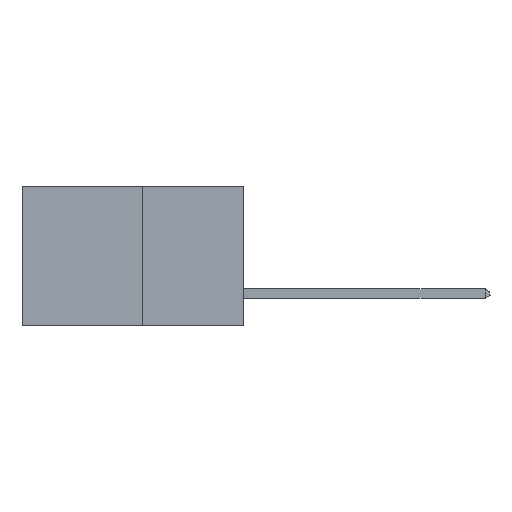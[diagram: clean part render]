
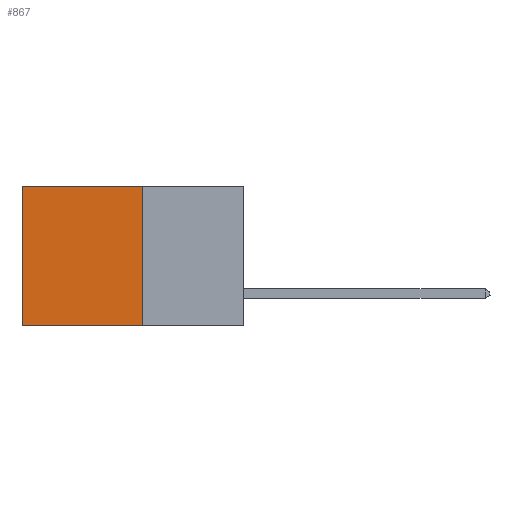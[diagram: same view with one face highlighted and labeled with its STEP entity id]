
A CAD part, left-side view. The second image highlights one B-rep face of the part: STEP entity #867.
In plain terms, the highlighted planar face has unit normal (-1, 0, 0).
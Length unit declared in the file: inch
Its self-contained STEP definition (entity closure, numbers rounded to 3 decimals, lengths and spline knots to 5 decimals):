
#722 = DIRECTION ( 'NONE',  ( 0., 1., 0. ) ) ;
#867 = ADVANCED_FACE ( 'NONE', ( #961 ), #1466, .F. ) ;
#955 = VECTOR ( 'NONE', #7400, 39.37008 ) ;
#961 = FACE_OUTER_BOUND ( 'NONE', #2803, .T. ) ;
#1003 = VECTOR ( 'NONE', #6351, 39.37008 ) ;
#1466 = PLANE ( 'NONE',  #8574 ) ;
#1635 = CARTESIAN_POINT ( 'NONE',  ( 0.277, 0.27, -0.37 ) ) ;
#1863 = DIRECTION ( 'NONE',  ( 0., 0., -1. ) ) ;
#1889 = DIRECTION ( 'NONE',  ( 1., 0., 0. ) ) ;
#1966 = CARTESIAN_POINT ( 'NONE',  ( 0.277, 0.27, 0. ) ) ;
#2147 = LINE ( 'NONE', #3714, #7726 ) ;
#2803 = EDGE_LOOP ( 'NONE', ( #3835, #4364, #6193, #6628 ) ) ;
#2861 = LINE ( 'NONE', #6359, #1003 ) ;
#2960 = VECTOR ( 'NONE', #722, 39.37008 ) ;
#3299 = LINE ( 'NONE', #6017, #955 ) ;
#3656 = DIRECTION ( 'NONE',  ( 0., 0., -1. ) ) ;
#3714 = CARTESIAN_POINT ( 'NONE',  ( 0.277, 0.59, -0.37 ) ) ;
#3835 = ORIENTED_EDGE ( 'NONE', *, *, #6360, .T. ) ;
#4311 = VERTEX_POINT ( 'NONE', #8397 ) ;
#4326 = CARTESIAN_POINT ( 'NONE',  ( 0.277, 0.27, -0.37 ) ) ;
#4364 = ORIENTED_EDGE ( 'NONE', *, *, #9088, .F. ) ;
#4849 = VERTEX_POINT ( 'NONE', #8983 ) ;
#5226 = EDGE_CURVE ( 'NONE', #6429, #8897, #2861, .T. ) ;
#6017 = CARTESIAN_POINT ( 'NONE',  ( 0.277, 0.27, -0.37 ) ) ;
#6193 = ORIENTED_EDGE ( 'NONE', *, *, #5226, .F. ) ;
#6351 = DIRECTION ( 'NONE',  ( 0., 0., -1. ) ) ;
#6359 = CARTESIAN_POINT ( 'NONE',  ( 0.277, 0.27, -0.37 ) ) ;
#6360 = EDGE_CURVE ( 'NONE', #4311, #4849, #2147, .T. ) ;
#6429 = VERTEX_POINT ( 'NONE', #1966 ) ;
#6628 = ORIENTED_EDGE ( 'NONE', *, *, #8462, .T. ) ;
#6654 = CARTESIAN_POINT ( 'NONE',  ( 0.277, 0.27, 0. ) ) ;
#7400 = DIRECTION ( 'NONE',  ( 0., 1., 0. ) ) ;
#7726 = VECTOR ( 'NONE', #3656, 39.37008 ) ;
#8397 = CARTESIAN_POINT ( 'NONE',  ( 0.277, 0.59, 0. ) ) ;
#8462 = EDGE_CURVE ( 'NONE', #6429, #4311, #8636, .T. ) ;
#8574 = AXIS2_PLACEMENT_3D ( 'NONE', #1635, #1889, #1863 ) ;
#8636 = LINE ( 'NONE', #6654, #2960 ) ;
#8897 = VERTEX_POINT ( 'NONE', #4326 ) ;
#8983 = CARTESIAN_POINT ( 'NONE',  ( 0.277, 0.59, -0.37 ) ) ;
#9088 = EDGE_CURVE ( 'NONE', #8897, #4849, #3299, .T. ) ;
